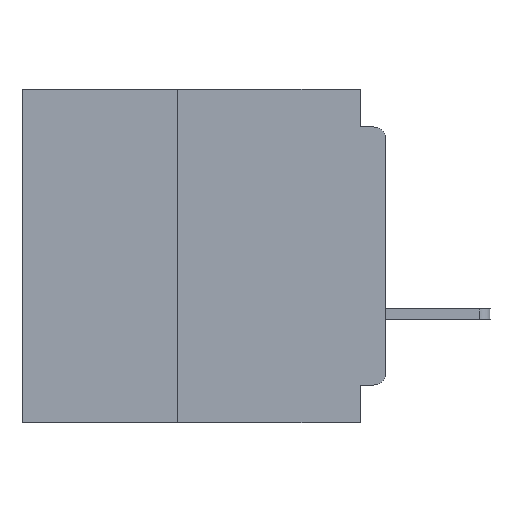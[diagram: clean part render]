
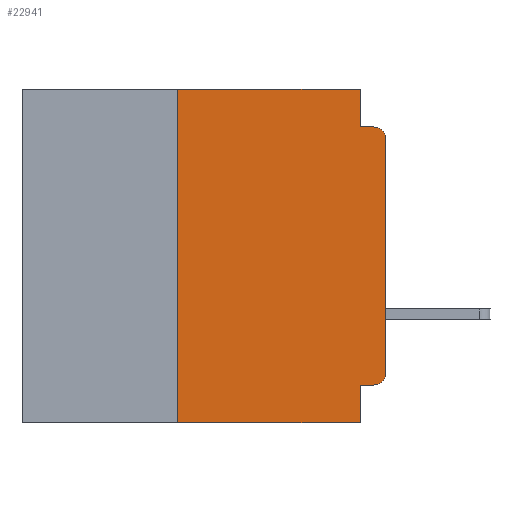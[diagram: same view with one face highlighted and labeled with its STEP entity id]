
A CAD part, left-side view. The second image highlights one B-rep face of the part: STEP entity #22941.
In plain terms, the highlighted planar face has unit normal (-1, 0, 0).
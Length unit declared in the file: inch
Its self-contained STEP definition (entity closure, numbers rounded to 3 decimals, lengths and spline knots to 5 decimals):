
#676 = EDGE_CURVE ( 'NONE', #36947, #55472, #28833, .T. ) ;
#1204 = DIRECTION ( 'NONE',  ( 0., 0., -1. ) ) ;
#1363 = ORIENTED_EDGE ( 'NONE', *, *, #56699, .F. ) ;
#1501 = EDGE_CURVE ( 'NONE', #7082, #54080, #21690, .T. ) ;
#2567 = DIRECTION ( 'NONE',  ( 0., 0., 1. ) ) ;
#3309 = ORIENTED_EDGE ( 'NONE', *, *, #22726, .T. ) ;
#4340 = CARTESIAN_POINT ( 'NONE',  ( 0., 0.015, -0.355 ) ) ;
#5053 = LINE ( 'NONE', #13532, #51914 ) ;
#6781 = ORIENTED_EDGE ( 'NONE', *, *, #31181, .T. ) ;
#7082 = VERTEX_POINT ( 'NONE', #39523 ) ;
#8483 = VERTEX_POINT ( 'NONE', #48775 ) ;
#9103 = VECTOR ( 'NONE', #2567, 39.37008 ) ;
#10676 = VECTOR ( 'NONE', #44360, 39.37008 ) ;
#11320 = ORIENTED_EDGE ( 'NONE', *, *, #17305, .F. ) ;
#12628 = CARTESIAN_POINT ( 'NONE',  ( 0., 0.437, -0.4 ) ) ;
#12646 = CARTESIAN_POINT ( 'NONE',  ( 0., 0., -0.045 ) ) ;
#13532 = CARTESIAN_POINT ( 'NONE',  ( 0., 0.25, -0.4 ) ) ;
#14748 = AXIS2_PLACEMENT_3D ( 'NONE', #36786, #18755, #50423 ) ;
#16735 = ORIENTED_EDGE ( 'NONE', *, *, #1501, .F. ) ;
#17305 = EDGE_CURVE ( 'NONE', #8483, #7082, #5053, .T. ) ;
#18224 = ORIENTED_EDGE ( 'NONE', *, *, #36129, .F. ) ;
#18755 = DIRECTION ( 'NONE',  ( 1., 0., 0. ) ) ;
#19072 = EDGE_CURVE ( 'NONE', #31480, #48745, #57498, .T. ) ;
#20580 = CARTESIAN_POINT ( 'NONE',  ( 0., 0.015, -0.34 ) ) ;
#20985 = CARTESIAN_POINT ( 'NONE',  ( 0., 0.031, 0. ) ) ;
#21258 = VECTOR ( 'NONE', #49403, 39.37008 ) ;
#21276 = ORIENTED_EDGE ( 'NONE', *, *, #47957, .F. ) ;
#21690 = LINE ( 'NONE', #39751, #56469 ) ;
#22726 = EDGE_CURVE ( 'NONE', #8483, #23311, #54868, .T. ) ;
#22941 = ADVANCED_FACE ( 'NONE', ( #47435 ), #45889, .F. ) ;
#23311 = VERTEX_POINT ( 'NONE', #57953 ) ;
#24047 = LINE ( 'NONE', #41316, #57404 ) ;
#24114 = LINE ( 'NONE', #44900, #21258 ) ;
#25157 = DIRECTION ( 'NONE',  ( 0., 0., -1. ) ) ;
#26261 = DIRECTION ( 'NONE',  ( 0., -1., 0. ) ) ;
#28573 = DIRECTION ( 'NONE',  ( -1., 0., 0. ) ) ;
#28833 = CIRCLE ( 'NONE', #54453, 0.015 ) ;
#29873 = CARTESIAN_POINT ( 'NONE',  ( 0., 0., 0. ) ) ;
#30075 = CIRCLE ( 'NONE', #42831, 0.015 ) ;
#30431 = ORIENTED_EDGE ( 'NONE', *, *, #34606, .T. ) ;
#30751 = VECTOR ( 'NONE', #58025, 39.37008 ) ;
#31181 = EDGE_CURVE ( 'NONE', #55472, #48562, #42452, .T. ) ;
#31480 = VERTEX_POINT ( 'NONE', #58968 ) ;
#33843 = ORIENTED_EDGE ( 'NONE', *, *, #676, .T. ) ;
#34606 = EDGE_CURVE ( 'NONE', #48562, #48745, #30075, .T. ) ;
#35154 = CARTESIAN_POINT ( 'NONE',  ( 0., 0., -0.34 ) ) ;
#36129 = EDGE_CURVE ( 'NONE', #54080, #31480, #54046, .T. ) ;
#36786 = CARTESIAN_POINT ( 'NONE',  ( 0., 0.437, 0. ) ) ;
#36947 = VERTEX_POINT ( 'NONE', #4340 ) ;
#39523 = CARTESIAN_POINT ( 'NONE',  ( 0., 0.25, 0. ) ) ;
#39751 = CARTESIAN_POINT ( 'NONE',  ( 0., 0.437, 0. ) ) ;
#40606 = VECTOR ( 'NONE', #48128, 39.37008 ) ;
#41214 = VERTEX_POINT ( 'NONE', #50444 ) ;
#41316 = CARTESIAN_POINT ( 'NONE',  ( 0., 0.031, -0.4 ) ) ;
#42452 = LINE ( 'NONE', #29873, #9103 ) ;
#42831 = AXIS2_PLACEMENT_3D ( 'NONE', #55694, #28573, #1204 ) ;
#42864 = EDGE_LOOP ( 'NONE', ( #6781, #30431, #50926, #18224, #16735, #11320, #3309, #1363, #21276, #33843 ) ) ;
#43447 = CARTESIAN_POINT ( 'NONE',  ( 0., 0.031, 0. ) ) ;
#44360 = DIRECTION ( 'NONE',  ( 0., -1., 0. ) ) ;
#44900 = CARTESIAN_POINT ( 'NONE',  ( 0., 0., -0.355 ) ) ;
#45854 = DIRECTION ( 'NONE',  ( 0., 0., -1. ) ) ;
#45889 = PLANE ( 'NONE',  #14748 ) ;
#46361 = CARTESIAN_POINT ( 'NONE',  ( 0., 0.015, -0.045 ) ) ;
#47435 = FACE_OUTER_BOUND ( 'NONE', #42864, .T. ) ;
#47957 = EDGE_CURVE ( 'NONE', #36947, #41214, #24114, .T. ) ;
#48128 = DIRECTION ( 'NONE',  ( 0., 0., -1. ) ) ;
#48562 = VERTEX_POINT ( 'NONE', #49341 ) ;
#48745 = VERTEX_POINT ( 'NONE', #46361 ) ;
#48775 = CARTESIAN_POINT ( 'NONE',  ( 0., 0.25, -0.4 ) ) ;
#49341 = CARTESIAN_POINT ( 'NONE',  ( 0., 0., -0.06 ) ) ;
#49403 = DIRECTION ( 'NONE',  ( 0., 1., 0. ) ) ;
#50423 = DIRECTION ( 'NONE',  ( 0., 0., -1. ) ) ;
#50444 = CARTESIAN_POINT ( 'NONE',  ( 0., 0.031, -0.355 ) ) ;
#50926 = ORIENTED_EDGE ( 'NONE', *, *, #19072, .F. ) ;
#51914 = VECTOR ( 'NONE', #58926, 39.37008 ) ;
#52277 = DIRECTION ( 'NONE',  ( -1., 0., 0. ) ) ;
#54046 = LINE ( 'NONE', #20985, #40606 ) ;
#54080 = VERTEX_POINT ( 'NONE', #43447 ) ;
#54453 = AXIS2_PLACEMENT_3D ( 'NONE', #20580, #52277, #25157 ) ;
#54868 = LINE ( 'NONE', #12628, #30751 ) ;
#55472 = VERTEX_POINT ( 'NONE', #35154 ) ;
#55694 = CARTESIAN_POINT ( 'NONE',  ( 0., 0.015, -0.06 ) ) ;
#56469 = VECTOR ( 'NONE', #26261, 39.37008 ) ;
#56699 = EDGE_CURVE ( 'NONE', #41214, #23311, #24047, .T. ) ;
#57404 = VECTOR ( 'NONE', #45854, 39.37008 ) ;
#57498 = LINE ( 'NONE', #12646, #10676 ) ;
#57953 = CARTESIAN_POINT ( 'NONE',  ( 0., 0.031, -0.4 ) ) ;
#58025 = DIRECTION ( 'NONE',  ( 0., -1., 0. ) ) ;
#58926 = DIRECTION ( 'NONE',  ( 0., 0., 1. ) ) ;
#58968 = CARTESIAN_POINT ( 'NONE',  ( 0., 0.031, -0.045 ) ) ;
